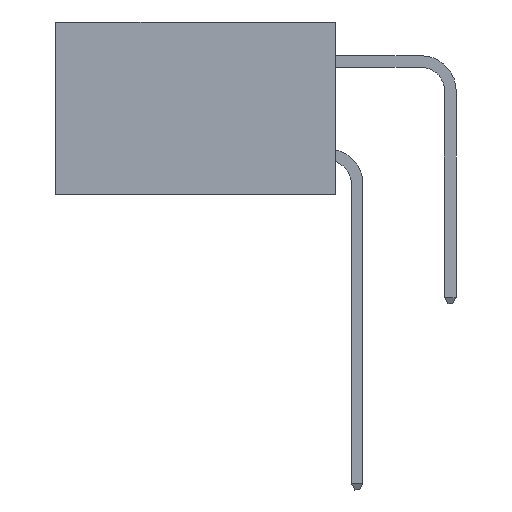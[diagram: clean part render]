
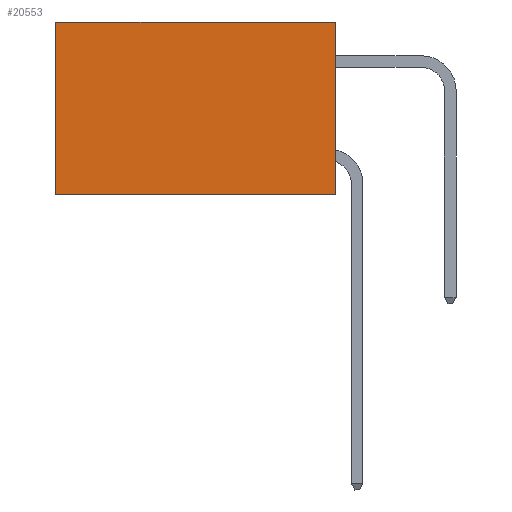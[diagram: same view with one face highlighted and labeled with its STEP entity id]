
A CAD part, left-side view. The second image highlights one B-rep face of the part: STEP entity #20553.
In plain terms, the highlighted planar face has unit normal (-1, 0, 0).
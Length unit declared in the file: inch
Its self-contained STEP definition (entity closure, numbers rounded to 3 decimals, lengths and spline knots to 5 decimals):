
#35 = AXIS2_PLACEMENT_3D ( 'NONE', #12105, #12376, #14393 ) ;
#463 = LINE ( 'NONE', #24915, #21324 ) ;
#2659 = EDGE_CURVE ( 'NONE', #20185, #8763, #463, .T. ) ;
#2772 = CARTESIAN_POINT ( 'NONE',  ( 0.2875, 0., 0. ) ) ;
#2874 = EDGE_CURVE ( 'NONE', #19041, #10313, #24989, .T. ) ;
#3278 = CARTESIAN_POINT ( 'NONE',  ( 0.2875, 0., -0.37 ) ) ;
#3660 = CARTESIAN_POINT ( 'NONE',  ( 0.2875, 0., 0. ) ) ;
#4113 = ORIENTED_EDGE ( 'NONE', *, *, #2874, .T. ) ;
#5405 = EDGE_CURVE ( 'NONE', #10313, #8763, #27224, .T. ) ;
#8763 = VERTEX_POINT ( 'NONE', #22753 ) ;
#9601 = CARTESIAN_POINT ( 'NONE',  ( 0.2875, 0.6, 0. ) ) ;
#10313 = VERTEX_POINT ( 'NONE', #9601 ) ;
#10940 = ORIENTED_EDGE ( 'NONE', *, *, #5405, .T. ) ;
#11508 = VECTOR ( 'NONE', #23233, 39.37008 ) ;
#12105 = CARTESIAN_POINT ( 'NONE',  ( 0.2875, 0., 0. ) ) ;
#12366 = EDGE_LOOP ( 'NONE', ( #10940, #19695, #15687, #4113 ) ) ;
#12376 = DIRECTION ( 'NONE',  ( 1., 0., 0. ) ) ;
#14247 = DIRECTION ( 'NONE',  ( 0., 1., 0. ) ) ;
#14393 = DIRECTION ( 'NONE',  ( 0., 0., -1. ) ) ;
#14820 = VECTOR ( 'NONE', #24872, 39.37008 ) ;
#15687 = ORIENTED_EDGE ( 'NONE', *, *, #27542, .F. ) ;
#16347 = PLANE ( 'NONE',  #35 ) ;
#18972 = FACE_OUTER_BOUND ( 'NONE', #12366, .T. ) ;
#19041 = VERTEX_POINT ( 'NONE', #27323 ) ;
#19695 = ORIENTED_EDGE ( 'NONE', *, *, #2659, .F. ) ;
#19988 = DIRECTION ( 'NONE',  ( 0., 0., -1. ) ) ;
#20185 = VERTEX_POINT ( 'NONE', #3278 ) ;
#20553 = ADVANCED_FACE ( 'NONE', ( #18972 ), #16347, .F. ) ;
#21324 = VECTOR ( 'NONE', #14247, 39.37008 ) ;
#21695 = LINE ( 'NONE', #2772, #22045 ) ;
#22045 = VECTOR ( 'NONE', #19988, 39.37008 ) ;
#22753 = CARTESIAN_POINT ( 'NONE',  ( 0.2875, 0.6, -0.37 ) ) ;
#23233 = DIRECTION ( 'NONE',  ( 0., 1., 0. ) ) ;
#24872 = DIRECTION ( 'NONE',  ( 0., 0., -1. ) ) ;
#24915 = CARTESIAN_POINT ( 'NONE',  ( 0.2875, 0., -0.37 ) ) ;
#24989 = LINE ( 'NONE', #3660, #11508 ) ;
#26860 = CARTESIAN_POINT ( 'NONE',  ( 0.2875, 0.6, 0. ) ) ;
#27224 = LINE ( 'NONE', #26860, #14820 ) ;
#27323 = CARTESIAN_POINT ( 'NONE',  ( 0.2875, 0., 0. ) ) ;
#27542 = EDGE_CURVE ( 'NONE', #19041, #20185, #21695, .T. ) ;
